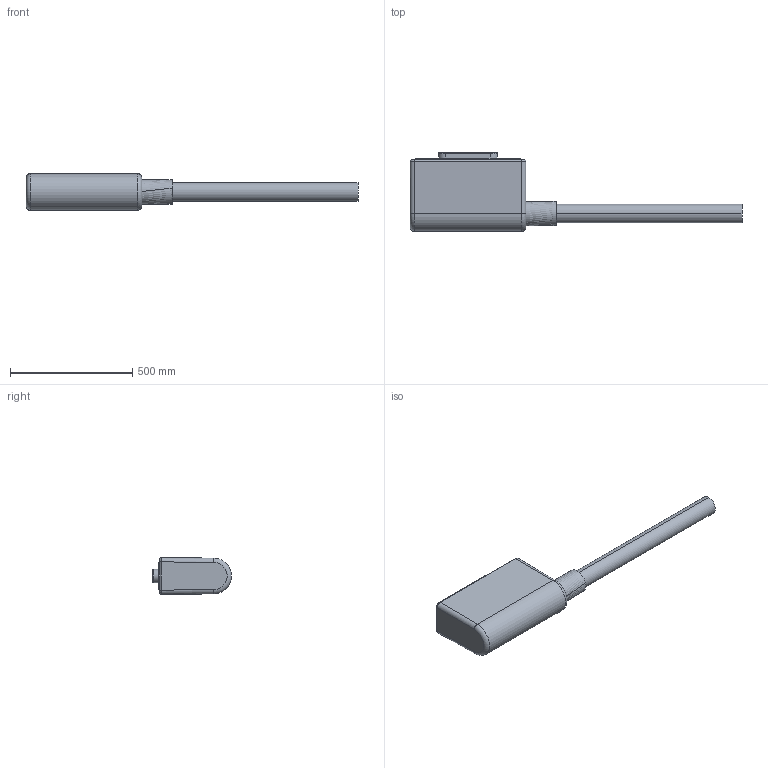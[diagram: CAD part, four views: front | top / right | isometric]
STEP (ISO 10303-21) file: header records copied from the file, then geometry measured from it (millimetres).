
FILE_DESCRIPTION (( 'STEP AP203' ), '1' );
FILE_NAME ('687B0521010120E.STEP', '2023-04-28T10:59:40', ( '' ), ( '' ), 'SwSTEP 2.0', 'SolidWorks 2020', '' );
FILE_SCHEMA (( 'CONFIG_CONTROL_DESIGN' ));
Length unit declared in the file: inch
Products named in the file (1): 687B0521010120E
Bounding box: 1360.17 x 323.34 x 151.51 mm (x, y, z)
Volume: 24450306.5 mm3; surface area: 714529.6 mm2
Topology: 1 solids, 1 shells, 89 faces, 185 edges, 112 vertices
Faces by surface type: cylinder 40, plane 25, torus 18, bspline 6
Entity records: 2754 total; most frequent: CARTESIAN_POINT 767, DIRECTION 435, ORIENTED_EDGE 370, EDGE_CURVE 185, AXIS2_PLACEMENT_3D 184, VERTEX_POINT 112, EDGE_LOOP 103, CIRCLE 100
